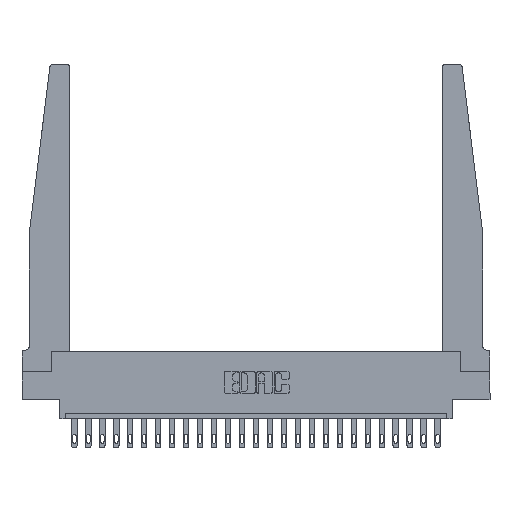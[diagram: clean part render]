
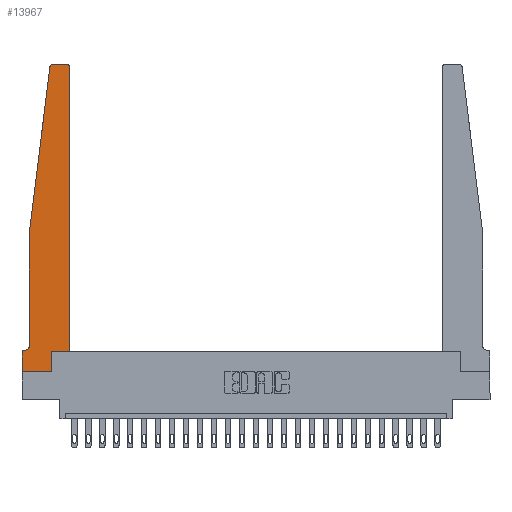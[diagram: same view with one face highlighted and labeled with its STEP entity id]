
A CAD part, top view. The second image highlights one B-rep face of the part: STEP entity #13967.
In plain terms, the highlighted planar face has unit normal (0, 0, 1).
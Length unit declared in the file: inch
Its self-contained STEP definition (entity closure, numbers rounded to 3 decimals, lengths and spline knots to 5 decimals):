
#178 = CARTESIAN_POINT ( 'NONE',  ( 0.25, 2.75, 0.37 ) ) ;
#580 = AXIS2_PLACEMENT_3D ( 'NONE', #5288, #5787, #12972 ) ;
#686 = DIRECTION ( 'NONE',  ( 0., 1., 0. ) ) ;
#1291 = VERTEX_POINT ( 'NONE', #17110 ) ;
#2330 = CARTESIAN_POINT ( 'NONE',  ( 0.425, 0.18, 0.37 ) ) ;
#2546 = EDGE_CURVE ( 'NONE', #15545, #19443, #21181, .T. ) ;
#2555 = LINE ( 'NONE', #19195, #10943 ) ;
#2664 = DIRECTION ( 'NONE',  ( 1., 0., 0. ) ) ;
#2869 = CARTESIAN_POINT ( 'NONE',  ( 0., 0., 0.37 ) ) ;
#2885 = ORIENTED_EDGE ( 'NONE', *, *, #15448, .T. ) ;
#2987 = CARTESIAN_POINT ( 'NONE',  ( 0.065, 1.25, 0.37 ) ) ;
#2996 = CARTESIAN_POINT ( 'NONE',  ( 0., 0., 0.37 ) ) ;
#3338 = EDGE_LOOP ( 'NONE', ( #23431, #23811, #7185, #16723, #20862, #11140, #12685, #12233, #2885, #12403, #15843, #4500 ) ) ;
#3490 = DIRECTION ( 'NONE',  ( 0., 0., 1. ) ) ;
#3524 = CARTESIAN_POINT ( 'NONE',  ( 0.24675, 2.72367, 0.37 ) ) ;
#3907 = FACE_OUTER_BOUND ( 'NONE', #3338, .T. ) ;
#4130 = VERTEX_POINT ( 'NONE', #2330 ) ;
#4500 = ORIENTED_EDGE ( 'NONE', *, *, #15219, .T. ) ;
#4805 = LINE ( 'NONE', #2987, #7980 ) ;
#5168 = DIRECTION ( 'NONE',  ( 0., -1., 0. ) ) ;
#5288 = CARTESIAN_POINT ( 'NONE',  ( 0.015, 0.2375, 0.37 ) ) ;
#5423 = VERTEX_POINT ( 'NONE', #16293 ) ;
#5730 = EDGE_CURVE ( 'NONE', #1291, #15509, #2555, .T. ) ;
#5787 = DIRECTION ( 'NONE',  ( 0., 0., -1. ) ) ;
#6059 = VERTEX_POINT ( 'NONE', #3524 ) ;
#6471 = VECTOR ( 'NONE', #19586, 39.37008 ) ;
#6516 = LINE ( 'NONE', #21093, #16037 ) ;
#6855 = LINE ( 'NONE', #19623, #9728 ) ;
#7185 = ORIENTED_EDGE ( 'NONE', *, *, #10350, .T. ) ;
#7490 = VERTEX_POINT ( 'NONE', #9160 ) ;
#7909 = DIRECTION ( 'NONE',  ( -1., 0., 0. ) ) ;
#7980 = VECTOR ( 'NONE', #10532, 39.37008 ) ;
#8068 = EDGE_CURVE ( 'NONE', #4130, #18040, #6516, .T. ) ;
#9160 = CARTESIAN_POINT ( 'NONE',  ( 0.2605, 0.18, 0.37 ) ) ;
#9631 = DIRECTION ( 'NONE',  ( 0., 0., 1. ) ) ;
#9728 = VECTOR ( 'NONE', #17910, 39.37008 ) ;
#10338 = CARTESIAN_POINT ( 'NONE',  ( 0.395, 2.72, 0.37 ) ) ;
#10350 = EDGE_CURVE ( 'NONE', #6059, #19073, #4805, .T. ) ;
#10532 = DIRECTION ( 'NONE',  ( -0.122, -0.992, 0. ) ) ;
#10808 = CIRCLE ( 'NONE', #23972, 0.03 ) ;
#10943 = VECTOR ( 'NONE', #7909, 39.37008 ) ;
#11140 = ORIENTED_EDGE ( 'NONE', *, *, #5730, .T. ) ;
#11205 = VECTOR ( 'NONE', #686, 39.37008 ) ;
#11808 = CARTESIAN_POINT ( 'NONE',  ( 0.27653, 2.72, 0.37 ) ) ;
#12203 = CARTESIAN_POINT ( 'NONE',  ( 0.425, 0.18, 0.37 ) ) ;
#12218 = VECTOR ( 'NONE', #5168, 39.37008 ) ;
#12233 = ORIENTED_EDGE ( 'NONE', *, *, #2546, .T. ) ;
#12263 = CARTESIAN_POINT ( 'NONE',  ( 0., 0.1875, 0.37 ) ) ;
#12376 = LINE ( 'NONE', #2869, #12218 ) ;
#12403 = ORIENTED_EDGE ( 'NONE', *, *, #13836, .T. ) ;
#12685 = ORIENTED_EDGE ( 'NONE', *, *, #22601, .T. ) ;
#12972 = DIRECTION ( 'NONE',  ( -1., 0., 0. ) ) ;
#13328 = CARTESIAN_POINT ( 'NONE',  ( 0.425, 2.72, 0.37 ) ) ;
#13830 = DIRECTION ( 'NONE',  ( 0., 1., 0. ) ) ;
#13836 = EDGE_CURVE ( 'NONE', #7490, #4130, #22003, .T. ) ;
#13967 = ADVANCED_FACE ( 'NONE', ( #3907 ), #14327, .T. ) ;
#14213 = DIRECTION ( 'NONE',  ( 0., 0., 1. ) ) ;
#14327 = PLANE ( 'NONE',  #16547 ) ;
#14444 = DIRECTION ( 'NONE',  ( 1., 0., 0. ) ) ;
#14968 = VECTOR ( 'NONE', #18291, 39.37008 ) ;
#14976 = EDGE_CURVE ( 'NONE', #5423, #6059, #16205, .T. ) ;
#15061 = LINE ( 'NONE', #18934, #11205 ) ;
#15219 = EDGE_CURVE ( 'NONE', #18040, #18257, #10808, .T. ) ;
#15448 = EDGE_CURVE ( 'NONE', #19443, #7490, #15061, .T. ) ;
#15509 = VERTEX_POINT ( 'NONE', #12263 ) ;
#15545 = VERTEX_POINT ( 'NONE', #2996 ) ;
#15695 = VECTOR ( 'NONE', #21057, 39.37008 ) ;
#15843 = ORIENTED_EDGE ( 'NONE', *, *, #8068, .T. ) ;
#16037 = VECTOR ( 'NONE', #13830, 39.37008 ) ;
#16118 = CIRCLE ( 'NONE', #580, 0.05 ) ;
#16205 = CIRCLE ( 'NONE', #23202, 0.03 ) ;
#16293 = CARTESIAN_POINT ( 'NONE',  ( 0.27653, 2.75, 0.37 ) ) ;
#16547 = AXIS2_PLACEMENT_3D ( 'NONE', #20130, #3490, #14444 ) ;
#16723 = ORIENTED_EDGE ( 'NONE', *, *, #17238, .T. ) ;
#17110 = CARTESIAN_POINT ( 'NONE',  ( 0.015, 0.1875, 0.37 ) ) ;
#17238 = EDGE_CURVE ( 'NONE', #19073, #23777, #6855, .T. ) ;
#17730 = DIRECTION ( 'NONE',  ( 1., 0., 0. ) ) ;
#17799 = CARTESIAN_POINT ( 'NONE',  ( 0.065, 1.25, 0.37 ) ) ;
#17910 = DIRECTION ( 'NONE',  ( 0., -1., 0. ) ) ;
#18004 = CARTESIAN_POINT ( 'NONE',  ( 0.2605, 0., 0.37 ) ) ;
#18040 = VERTEX_POINT ( 'NONE', #13328 ) ;
#18257 = VERTEX_POINT ( 'NONE', #21743 ) ;
#18291 = DIRECTION ( 'NONE',  ( -1., 0., 0. ) ) ;
#18661 = LINE ( 'NONE', #178, #14968 ) ;
#18934 = CARTESIAN_POINT ( 'NONE',  ( 0.2605, 0.18, 0.37 ) ) ;
#19073 = VERTEX_POINT ( 'NONE', #17799 ) ;
#19195 = CARTESIAN_POINT ( 'NONE',  ( 0.065, 0.1875, 0.37 ) ) ;
#19368 = CARTESIAN_POINT ( 'NONE',  ( 0., 0., 0.37 ) ) ;
#19443 = VERTEX_POINT ( 'NONE', #18004 ) ;
#19586 = DIRECTION ( 'NONE',  ( 1., 0., 0. ) ) ;
#19623 = CARTESIAN_POINT ( 'NONE',  ( 0.065, 1.25, 0.37 ) ) ;
#20130 = CARTESIAN_POINT ( 'NONE',  ( 0., 0.1875, 0.37 ) ) ;
#20862 = ORIENTED_EDGE ( 'NONE', *, *, #23980, .T. ) ;
#21057 = DIRECTION ( 'NONE',  ( 1., 0., 0. ) ) ;
#21093 = CARTESIAN_POINT ( 'NONE',  ( 0.425, 0.18, 0.37 ) ) ;
#21181 = LINE ( 'NONE', #19368, #15695 ) ;
#21336 = CARTESIAN_POINT ( 'NONE',  ( 0.065, 0.2375, 0.37 ) ) ;
#21743 = CARTESIAN_POINT ( 'NONE',  ( 0.395, 2.75, 0.37 ) ) ;
#22003 = LINE ( 'NONE', #12203, #6471 ) ;
#22601 = EDGE_CURVE ( 'NONE', #15509, #15545, #12376, .T. ) ;
#23202 = AXIS2_PLACEMENT_3D ( 'NONE', #11808, #9631, #2664 ) ;
#23431 = ORIENTED_EDGE ( 'NONE', *, *, #23954, .T. ) ;
#23777 = VERTEX_POINT ( 'NONE', #21336 ) ;
#23811 = ORIENTED_EDGE ( 'NONE', *, *, #14976, .T. ) ;
#23954 = EDGE_CURVE ( 'NONE', #18257, #5423, #18661, .T. ) ;
#23972 = AXIS2_PLACEMENT_3D ( 'NONE', #10338, #14213, #17730 ) ;
#23980 = EDGE_CURVE ( 'NONE', #23777, #1291, #16118, .T. ) ;
